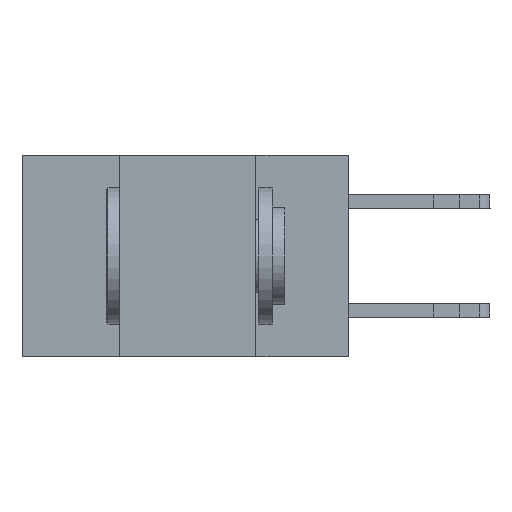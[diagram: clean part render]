
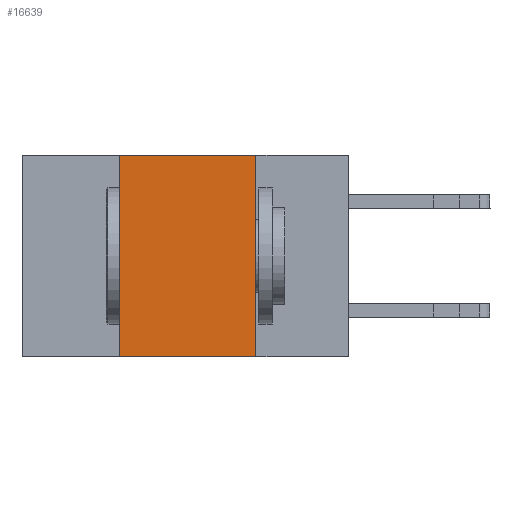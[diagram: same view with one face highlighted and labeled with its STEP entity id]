
A CAD part, left-side view. The second image highlights one B-rep face of the part: STEP entity #16639.
In plain terms, the highlighted planar face has unit normal (-1, 0, 0).
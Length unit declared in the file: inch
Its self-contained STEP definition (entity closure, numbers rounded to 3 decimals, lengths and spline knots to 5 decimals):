
#75 = DIRECTION ( 'NONE',  ( 0., 0., -1. ) ) ;
#584 = DIRECTION ( 'NONE',  ( 0., 0., 1. ) ) ;
#1441 = VERTEX_POINT ( 'NONE', #4310 ) ;
#2128 = CARTESIAN_POINT ( 'NONE',  ( 0., 0.42, -0.37 ) ) ;
#3108 = VERTEX_POINT ( 'NONE', #4003 ) ;
#3811 = DIRECTION ( 'NONE',  ( 0., -1., 0. ) ) ;
#4003 = CARTESIAN_POINT ( 'NONE',  ( 0., 0.42, 0. ) ) ;
#4310 = CARTESIAN_POINT ( 'NONE',  ( 0., 0.17, -0.37 ) ) ;
#4818 = VERTEX_POINT ( 'NONE', #5306 ) ;
#5236 = LINE ( 'NONE', #11143, #18963 ) ;
#5306 = CARTESIAN_POINT ( 'NONE',  ( 0., 0.17, 0. ) ) ;
#5332 = VECTOR ( 'NONE', #14597, 39.37008 ) ;
#5708 = CARTESIAN_POINT ( 'NONE',  ( 0., 0.6, 0. ) ) ;
#6269 = EDGE_CURVE ( 'NONE', #13583, #3108, #9350, .T. ) ;
#6984 = EDGE_CURVE ( 'NONE', #13583, #1441, #5236, .T. ) ;
#7185 = FACE_OUTER_BOUND ( 'NONE', #10664, .T. ) ;
#7698 = CARTESIAN_POINT ( 'NONE',  ( 0., 0.42, -0.37 ) ) ;
#8040 = LINE ( 'NONE', #17078, #13335 ) ;
#8194 = VECTOR ( 'NONE', #584, 39.37008 ) ;
#8450 = AXIS2_PLACEMENT_3D ( 'NONE', #13067, #14914, #75 ) ;
#8717 = LINE ( 'NONE', #5708, #5332 ) ;
#9150 = ORIENTED_EDGE ( 'NONE', *, *, #6269, .F. ) ;
#9350 = LINE ( 'NONE', #2128, #8194 ) ;
#10664 = EDGE_LOOP ( 'NONE', ( #11725, #15912, #9150, #15582 ) ) ;
#11143 = CARTESIAN_POINT ( 'NONE',  ( 0., 0.6, -0.37 ) ) ;
#11725 = ORIENTED_EDGE ( 'NONE', *, *, #17363, .F. ) ;
#13067 = CARTESIAN_POINT ( 'NONE',  ( 0., 0.6, 0. ) ) ;
#13335 = VECTOR ( 'NONE', #14002, 39.37008 ) ;
#13583 = VERTEX_POINT ( 'NONE', #7698 ) ;
#14002 = DIRECTION ( 'NONE',  ( 0., 0., -1. ) ) ;
#14597 = DIRECTION ( 'NONE',  ( 0., -1., 0. ) ) ;
#14914 = DIRECTION ( 'NONE',  ( 1., 0., 0. ) ) ;
#15582 = ORIENTED_EDGE ( 'NONE', *, *, #6984, .T. ) ;
#15605 = EDGE_CURVE ( 'NONE', #3108, #4818, #8717, .T. ) ;
#15912 = ORIENTED_EDGE ( 'NONE', *, *, #15605, .F. ) ;
#16639 = ADVANCED_FACE ( 'NONE', ( #7185 ), #17694, .F. ) ;
#17078 = CARTESIAN_POINT ( 'NONE',  ( 0., 0.17, -0.37 ) ) ;
#17363 = EDGE_CURVE ( 'NONE', #4818, #1441, #8040, .T. ) ;
#17694 = PLANE ( 'NONE',  #8450 ) ;
#18963 = VECTOR ( 'NONE', #3811, 39.37008 ) ;
